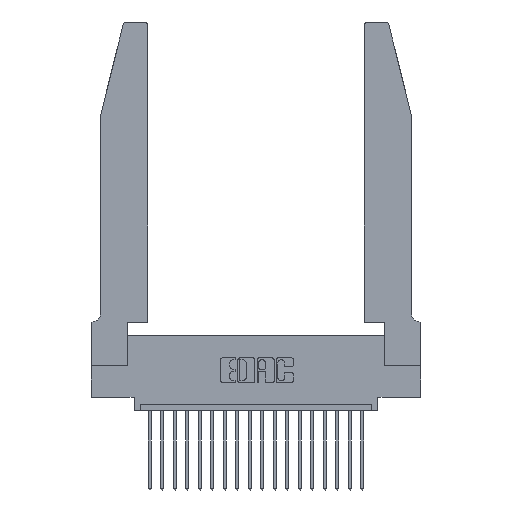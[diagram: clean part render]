
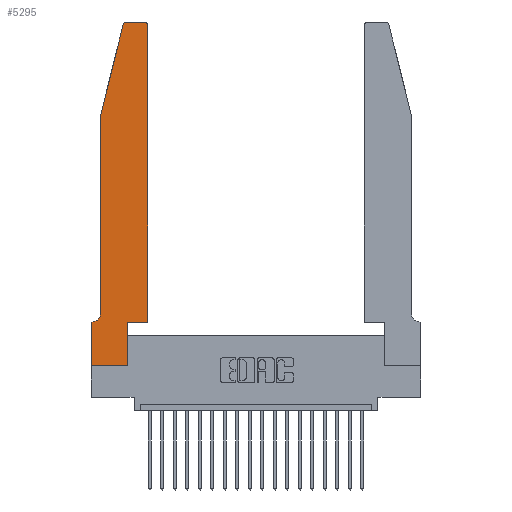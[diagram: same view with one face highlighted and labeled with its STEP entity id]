
A CAD part, top view. The second image highlights one B-rep face of the part: STEP entity #5295.
In plain terms, the highlighted planar face has unit normal (0, 0, 1).
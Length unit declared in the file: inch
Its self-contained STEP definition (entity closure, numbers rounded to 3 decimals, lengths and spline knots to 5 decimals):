
#261 = DIRECTION ( 'NONE',  ( 1., 0., 0. ) ) ;
#300 = AXIS2_PLACEMENT_3D ( 'NONE', #18089, #16768, #13381 ) ;
#311 = ORIENTED_EDGE ( 'NONE', *, *, #9327, .T. ) ;
#382 = LINE ( 'NONE', #7532, #4338 ) ;
#622 = EDGE_CURVE ( 'NONE', #10564, #20295, #4991, .T. ) ;
#926 = VERTEX_POINT ( 'NONE', #16709 ) ;
#1002 = EDGE_CURVE ( 'NONE', #18136, #5159, #10485, .T. ) ;
#1214 = CIRCLE ( 'NONE', #1556, 0.07 ) ;
#1297 = CARTESIAN_POINT ( 'NONE',  ( 0., 0., 0.37 ) ) ;
#1556 = AXIS2_PLACEMENT_3D ( 'NONE', #15270, #11845, #16806 ) ;
#2251 = EDGE_CURVE ( 'NONE', #5559, #5148, #5173, .T. ) ;
#2287 = LINE ( 'NONE', #20382, #7535 ) ;
#2336 = EDGE_CURVE ( 'NONE', #20295, #5559, #19833, .T. ) ;
#2401 = DIRECTION ( 'NONE',  ( 1., 0., 0. ) ) ;
#2437 = CARTESIAN_POINT ( 'NONE',  ( 0., 0., 0.37 ) ) ;
#2558 = DIRECTION ( 'NONE',  ( 0., -1., 0. ) ) ;
#3587 = DIRECTION ( 'NONE',  ( -1., 0., 0. ) ) ;
#3654 = ORIENTED_EDGE ( 'NONE', *, *, #12179, .T. ) ;
#3735 = VECTOR ( 'NONE', #11130, 39.37008 ) ;
#3874 = CARTESIAN_POINT ( 'NONE',  ( 0.4505, 0.35, 0.37 ) ) ;
#4241 = CARTESIAN_POINT ( 'NONE',  ( 0., 0.35, 0.37 ) ) ;
#4338 = VECTOR ( 'NONE', #2558, 39.37008 ) ;
#4359 = LINE ( 'NONE', #4551, #7742 ) ;
#4394 = VECTOR ( 'NONE', #3587, 39.37008 ) ;
#4529 = CARTESIAN_POINT ( 'NONE',  ( 0.4505, 0.35, 0.37 ) ) ;
#4538 = VERTEX_POINT ( 'NONE', #9370 ) ;
#4551 = CARTESIAN_POINT ( 'NONE',  ( 0., 0., 0.37 ) ) ;
#4991 = CIRCLE ( 'NONE', #19938, 0.03 ) ;
#5047 = CARTESIAN_POINT ( 'NONE',  ( 0.25487, 2.72718, 0.37 ) ) ;
#5148 = VERTEX_POINT ( 'NONE', #5047 ) ;
#5159 = VERTEX_POINT ( 'NONE', #3874 ) ;
#5173 = CIRCLE ( 'NONE', #300, 0.03 ) ;
#5220 = ORIENTED_EDGE ( 'NONE', *, *, #2336, .T. ) ;
#5295 = ADVANCED_FACE ( 'NONE', ( #6094 ), #5413, .T. ) ;
#5413 = PLANE ( 'NONE',  #21237 ) ;
#5414 = DIRECTION ( 'NONE',  ( 0., 0., 1. ) ) ;
#5559 = VERTEX_POINT ( 'NONE', #14521 ) ;
#5701 = ORIENTED_EDGE ( 'NONE', *, *, #12117, .T. ) ;
#5707 = DIRECTION ( 'NONE',  ( 0., 0., 1. ) ) ;
#6094 = FACE_OUTER_BOUND ( 'NONE', #17868, .T. ) ;
#7481 = VECTOR ( 'NONE', #8328, 39.37008 ) ;
#7532 = CARTESIAN_POINT ( 'NONE',  ( 0.0755, 2., 0.37 ) ) ;
#7535 = VECTOR ( 'NONE', #10388, 39.37008 ) ;
#7742 = VECTOR ( 'NONE', #16390, 39.37008 ) ;
#8096 = CARTESIAN_POINT ( 'NONE',  ( 0.0755, 2., 0.37 ) ) ;
#8162 = LINE ( 'NONE', #1297, #3735 ) ;
#8328 = DIRECTION ( 'NONE',  ( -0.239, -0.971, 0. ) ) ;
#8702 = VERTEX_POINT ( 'NONE', #2437 ) ;
#8750 = LINE ( 'NONE', #17277, #19764 ) ;
#9129 = EDGE_CURVE ( 'NONE', #5148, #4538, #11152, .T. ) ;
#9327 = EDGE_CURVE ( 'NONE', #8702, #19340, #4359, .T. ) ;
#9370 = CARTESIAN_POINT ( 'NONE',  ( 0.0755, 2., 0.37 ) ) ;
#9704 = DIRECTION ( 'NONE',  ( 1., 0., 0. ) ) ;
#10191 = CARTESIAN_POINT ( 'NONE',  ( 0.2605, 2.75, 0.37 ) ) ;
#10388 = DIRECTION ( 'NONE',  ( 0., 1., 0. ) ) ;
#10485 = LINE ( 'NONE', #4529, #18604 ) ;
#10564 = VERTEX_POINT ( 'NONE', #16824 ) ;
#11130 = DIRECTION ( 'NONE',  ( 0., -1., 0. ) ) ;
#11152 = LINE ( 'NONE', #8096, #7481 ) ;
#11523 = CARTESIAN_POINT ( 'NONE',  ( 0.0055, 0.35, 0.37 ) ) ;
#11845 = DIRECTION ( 'NONE',  ( 0., 0., -1. ) ) ;
#11850 = CARTESIAN_POINT ( 'NONE',  ( 0.4505, 0.35, 0.37 ) ) ;
#11872 = VERTEX_POINT ( 'NONE', #19623 ) ;
#12117 = EDGE_CURVE ( 'NONE', #19340, #18136, #2287, .T. ) ;
#12179 = EDGE_CURVE ( 'NONE', #11872, #16308, #1214, .T. ) ;
#12274 = ORIENTED_EDGE ( 'NONE', *, *, #2251, .T. ) ;
#12416 = CARTESIAN_POINT ( 'NONE',  ( 0.2865, 0., 0.37 ) ) ;
#13381 = DIRECTION ( 'NONE',  ( 1., 0., 0. ) ) ;
#13488 = EDGE_CURVE ( 'NONE', #4538, #11872, #382, .T. ) ;
#13595 = CARTESIAN_POINT ( 'NONE',  ( 0.2865, 0.35, 0.37 ) ) ;
#13609 = ORIENTED_EDGE ( 'NONE', *, *, #9129, .T. ) ;
#14521 = CARTESIAN_POINT ( 'NONE',  ( 0.284, 2.75, 0.37 ) ) ;
#14580 = EDGE_CURVE ( 'NONE', #16308, #926, #8750, .T. ) ;
#14821 = ORIENTED_EDGE ( 'NONE', *, *, #1002, .T. ) ;
#15270 = CARTESIAN_POINT ( 'NONE',  ( 0.0055, 0.42, 0.37 ) ) ;
#15433 = CARTESIAN_POINT ( 'NONE',  ( 0.4205, 2.72, 0.37 ) ) ;
#15517 = LINE ( 'NONE', #11850, #19469 ) ;
#15563 = ORIENTED_EDGE ( 'NONE', *, *, #13488, .T. ) ;
#15831 = ORIENTED_EDGE ( 'NONE', *, *, #622, .T. ) ;
#15897 = EDGE_CURVE ( 'NONE', #926, #8702, #8162, .T. ) ;
#16070 = ORIENTED_EDGE ( 'NONE', *, *, #14580, .T. ) ;
#16308 = VERTEX_POINT ( 'NONE', #11523 ) ;
#16390 = DIRECTION ( 'NONE',  ( 1., 0., 0. ) ) ;
#16709 = CARTESIAN_POINT ( 'NONE',  ( 0., 0.35, 0.37 ) ) ;
#16768 = DIRECTION ( 'NONE',  ( 0., 0., 1. ) ) ;
#16806 = DIRECTION ( 'NONE',  ( -1., 0., 0. ) ) ;
#16824 = CARTESIAN_POINT ( 'NONE',  ( 0.4505, 2.72, 0.37 ) ) ;
#17056 = DIRECTION ( 'NONE',  ( -1., 0., 0. ) ) ;
#17277 = CARTESIAN_POINT ( 'NONE',  ( 0.0755, 0.35, 0.37 ) ) ;
#17864 = ORIENTED_EDGE ( 'NONE', *, *, #20396, .T. ) ;
#17868 = EDGE_LOOP ( 'NONE', ( #5220, #12274, #13609, #15563, #3654, #16070, #20065, #311, #5701, #14821, #17864, #15831 ) ) ;
#18089 = CARTESIAN_POINT ( 'NONE',  ( 0.284, 2.72, 0.37 ) ) ;
#18136 = VERTEX_POINT ( 'NONE', #13595 ) ;
#18604 = VECTOR ( 'NONE', #9704, 39.37008 ) ;
#19340 = VERTEX_POINT ( 'NONE', #12416 ) ;
#19469 = VECTOR ( 'NONE', #20238, 39.37008 ) ;
#19623 = CARTESIAN_POINT ( 'NONE',  ( 0.0755, 0.42, 0.37 ) ) ;
#19764 = VECTOR ( 'NONE', #17056, 39.37008 ) ;
#19833 = LINE ( 'NONE', #10191, #4394 ) ;
#19938 = AXIS2_PLACEMENT_3D ( 'NONE', #15433, #5414, #261 ) ;
#20065 = ORIENTED_EDGE ( 'NONE', *, *, #15897, .T. ) ;
#20238 = DIRECTION ( 'NONE',  ( 0., 1., 0. ) ) ;
#20295 = VERTEX_POINT ( 'NONE', #21331 ) ;
#20382 = CARTESIAN_POINT ( 'NONE',  ( 0.2865, 0.35, 0.37 ) ) ;
#20396 = EDGE_CURVE ( 'NONE', #5159, #10564, #15517, .T. ) ;
#21237 = AXIS2_PLACEMENT_3D ( 'NONE', #4241, #5707, #2401 ) ;
#21331 = CARTESIAN_POINT ( 'NONE',  ( 0.4205, 2.75, 0.37 ) ) ;
